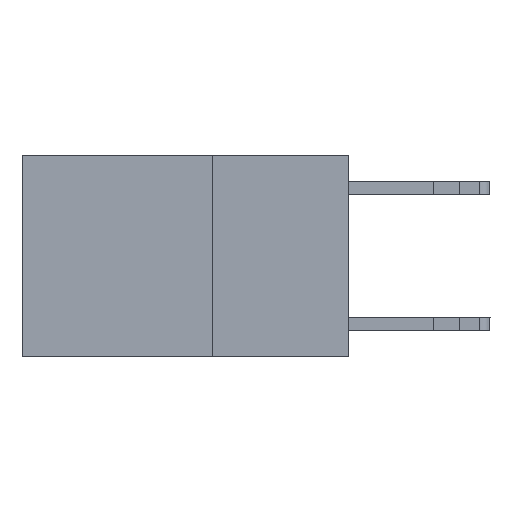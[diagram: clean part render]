
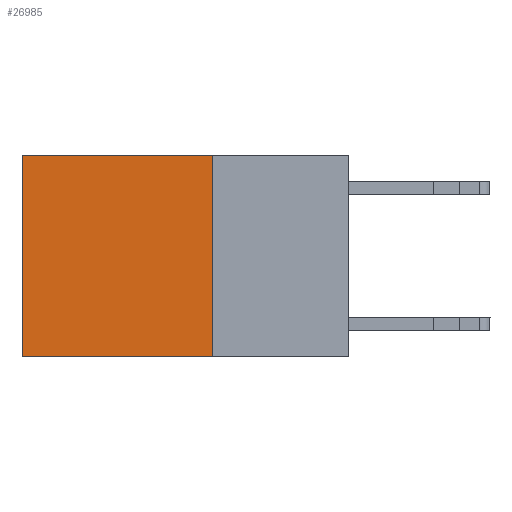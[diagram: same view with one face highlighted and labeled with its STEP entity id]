
A CAD part, left-side view. The second image highlights one B-rep face of the part: STEP entity #26985.
In plain terms, the highlighted planar face has unit normal (-1, 0, 0).
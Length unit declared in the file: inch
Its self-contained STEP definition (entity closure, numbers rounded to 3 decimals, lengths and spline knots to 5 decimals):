
#227 = ORIENTED_EDGE ( 'NONE', *, *, #8780, .F. ) ;
#1344 = EDGE_CURVE ( 'NONE', #4312, #14381, #23802, .T. ) ;
#1645 = VECTOR ( 'NONE', #9368, 39.37008 ) ;
#1730 = LINE ( 'NONE', #9487, #1645 ) ;
#2229 = VERTEX_POINT ( 'NONE', #5130 ) ;
#2889 = ORIENTED_EDGE ( 'NONE', *, *, #24683, .T. ) ;
#4134 = VECTOR ( 'NONE', #23381, 39.37008 ) ;
#4303 = LINE ( 'NONE', #21349, #4134 ) ;
#4312 = VERTEX_POINT ( 'NONE', #21884 ) ;
#4515 = PLANE ( 'NONE',  #5320 ) ;
#5130 = CARTESIAN_POINT ( 'NONE',  ( 0.2625, 0.25, 0. ) ) ;
#5320 = AXIS2_PLACEMENT_3D ( 'NONE', #21614, #8908, #23616 ) ;
#8780 = EDGE_CURVE ( 'NONE', #16257, #14381, #1730, .T. ) ;
#8908 = DIRECTION ( 'NONE',  ( 1., 0., 0. ) ) ;
#8910 = FACE_OUTER_BOUND ( 'NONE', #13688, .T. ) ;
#9368 = DIRECTION ( 'NONE',  ( 0., 1., 0. ) ) ;
#9487 = CARTESIAN_POINT ( 'NONE',  ( 0.2625, 0.25, -0.37 ) ) ;
#11146 = CARTESIAN_POINT ( 'NONE',  ( 0.2625, 0.6, -0.37 ) ) ;
#11779 = LINE ( 'NONE', #23774, #12184 ) ;
#12184 = VECTOR ( 'NONE', #13310, 39.37008 ) ;
#12202 = CARTESIAN_POINT ( 'NONE',  ( 0.2625, 0.25, -0.37 ) ) ;
#13310 = DIRECTION ( 'NONE',  ( 0., 0., -1. ) ) ;
#13671 = ORIENTED_EDGE ( 'NONE', *, *, #1344, .T. ) ;
#13688 = EDGE_LOOP ( 'NONE', ( #13671, #227, #17888, #2889 ) ) ;
#14381 = VERTEX_POINT ( 'NONE', #11146 ) ;
#16257 = VERTEX_POINT ( 'NONE', #12202 ) ;
#17888 = ORIENTED_EDGE ( 'NONE', *, *, #25455, .F. ) ;
#21349 = CARTESIAN_POINT ( 'NONE',  ( 0.2625, 0.25, 0. ) ) ;
#21614 = CARTESIAN_POINT ( 'NONE',  ( 0.2625, 0.25, 0. ) ) ;
#21884 = CARTESIAN_POINT ( 'NONE',  ( 0.2625, 0.6, 0. ) ) ;
#23381 = DIRECTION ( 'NONE',  ( 0., 1., 0. ) ) ;
#23616 = DIRECTION ( 'NONE',  ( 0., 0., -1. ) ) ;
#23671 = VECTOR ( 'NONE', #26909, 39.37008 ) ;
#23774 = CARTESIAN_POINT ( 'NONE',  ( 0.2625, 0.25, 0. ) ) ;
#23802 = LINE ( 'NONE', #26919, #23671 ) ;
#24683 = EDGE_CURVE ( 'NONE', #2229, #4312, #4303, .T. ) ;
#25455 = EDGE_CURVE ( 'NONE', #2229, #16257, #11779, .T. ) ;
#26909 = DIRECTION ( 'NONE',  ( 0., 0., -1. ) ) ;
#26919 = CARTESIAN_POINT ( 'NONE',  ( 0.2625, 0.6, 0. ) ) ;
#26985 = ADVANCED_FACE ( 'NONE', ( #8910 ), #4515, .F. ) ;
